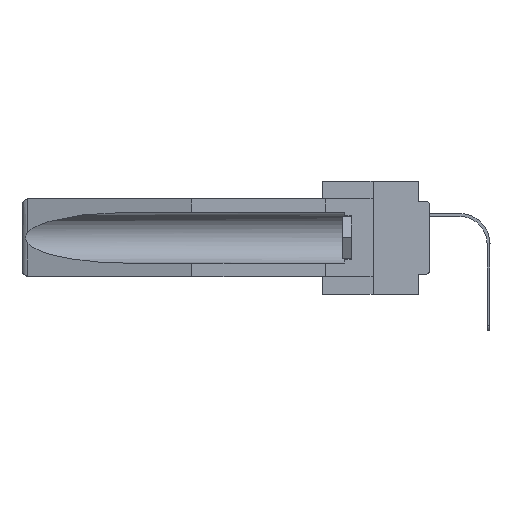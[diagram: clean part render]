
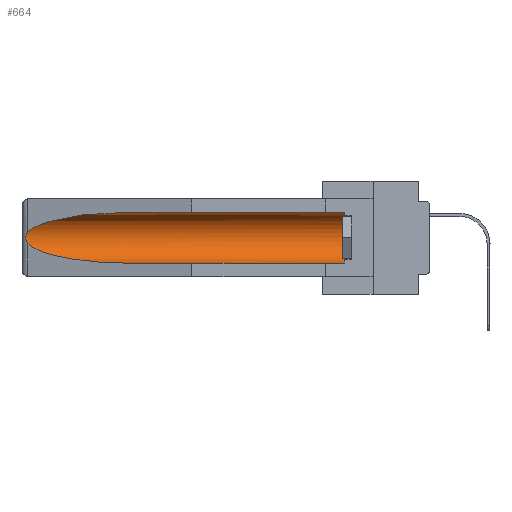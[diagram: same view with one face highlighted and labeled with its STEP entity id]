
A CAD part, left-side view. The second image highlights one B-rep face of the part: STEP entity #664.
In plain terms, the highlighted cylindrical face has radius 2.857 mm (diameter 5.715 mm), a partial arc.
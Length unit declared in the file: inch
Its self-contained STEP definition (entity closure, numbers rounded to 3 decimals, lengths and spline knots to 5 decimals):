
#32 = CARTESIAN_POINT ( 'NONE',  ( 0.155, 1.07973, -0.284 ) ) ;
#664 = ADVANCED_FACE ( 'NONE', ( #27719 ), #1454, .F. ) ;
#842 = CIRCLE ( 'NONE', #33947, 0.1125 ) ;
#1454 = CYLINDRICAL_SURFACE ( 'NONE', #13421, 0.1125 ) ;
#1551 = CARTESIAN_POINT ( 'NONE',  ( 0.26655, 1.53094, -0.18657 ) ) ;
#1882 = CARTESIAN_POINT ( 'NONE',  ( 0.2673, 1.53269, -0.17917 ) ) ;
#3863 = EDGE_CURVE ( 'NONE', #22414, #10565, #8504, .T. ) ;
#3926 = VERTEX_POINT ( 'NONE', #30765 ) ;
#4360 = CARTESIAN_POINT ( 'NONE',  ( 0.21114, 1.30732, -0.059 ) ) ;
#4873 = EDGE_CURVE ( 'NONE', #20516, #3926, #15691, .T. ) ;
#5853 = DIRECTION ( 'NONE',  ( 0., 0., 1. ) ) ;
#6757 = CARTESIAN_POINT ( 'NONE',  ( 0.2675, 1.53308, -0.16763 ) ) ;
#7112 = CARTESIAN_POINT ( 'NONE',  ( 0.155, 1.07973, -0.059 ) ) ;
#7717 = B_SPLINE_CURVE_WITH_KNOTS ( 'NONE', 3,
 ( #20226, #15039, #28470, #30579, #6757, #22804, #1882, #1551, #15196, #12118 ),
 .UNSPECIFIED., .F., .F.,
 ( 4, 2, 2, 2, 4 ),
 ( 0., 0.00029, 0.00058, 0.00087, 0.00117 ),
 .UNSPECIFIED. ) ;
#8137 = CARTESIAN_POINT ( 'NONE',  ( 0.155, 1.07973, -0.059 ) ) ;
#8504 = LINE ( 'NONE', #21622, #13854 ) ;
#8625 = LINE ( 'NONE', #24515, #11952 ) ;
#8847 = ORIENTED_EDGE ( 'NONE', *, *, #4873, .T. ) ;
#9611 = CARTESIAN_POINT ( 'NONE',  ( 0.155, -0.30754, -0.1715 ) ) ;
#10565 = VERTEX_POINT ( 'NONE', #8137 ) ;
#10967 = CARTESIAN_POINT ( 'NONE',  ( 0.155, 0.126, -0.059 ) ) ;
#11381 = DIRECTION ( 'NONE',  ( 0., 1., 0. ) ) ;
#11942 = EDGE_CURVE ( 'NONE', #20156, #20516, #7717, .T. ) ;
#11952 = VECTOR ( 'NONE', #11381, 39.37008 ) ;
#12118 = CARTESIAN_POINT ( 'NONE',  ( 0.26537, 1.52718, -0.19328 ) ) ;
#12153 = EDGE_CURVE ( 'NONE', #31671, #22414, #842, .T. ) ;
#12718 = CARTESIAN_POINT ( 'NONE',  ( 0.26537, 1.52718, -0.14972 ) ) ;
#12835 = CARTESIAN_POINT ( 'NONE',  ( 0.26537, 1.52718, -0.19328 ) ) ;
#13421 = AXIS2_PLACEMENT_3D ( 'NONE', #9611, #22378, #32929 ) ;
#13431 = EDGE_CURVE ( 'NONE', #31671, #3926, #8625, .T. ) ;
#13507 = CARTESIAN_POINT ( 'NONE',  ( 0.25451, 1.48313, -0.24835 ) ) ;
#13854 = VECTOR ( 'NONE', #14033, 39.37008 ) ;
#14033 = DIRECTION ( 'NONE',  ( 0., 1., 0. ) ) ;
#15039 = CARTESIAN_POINT ( 'NONE',  ( 0.26597, 1.52961, -0.15275 ) ) ;
#15196 = CARTESIAN_POINT ( 'NONE',  ( 0.26597, 1.5296, -0.19026 ) ) ;
#15691 =( BOUNDED_CURVE ( )  B_SPLINE_CURVE ( 3, ( #12835, #13507, #29037, #32 ),
 .UNSPECIFIED., .F., .F. ) 
 B_SPLINE_CURVE_WITH_KNOTS ( ( 4, 4 ),
 ( 0.1948, 1.5708 ),
 .UNSPECIFIED. ) 
 CURVE ( )  GEOMETRIC_REPRESENTATION_ITEM ( )  RATIONAL_B_SPLINE_CURVE ( ( 1., 0.848, 0.848, 1. ) ) 
 REPRESENTATION_ITEM ( '' )  );
#16050 = ORIENTED_EDGE ( 'NONE', *, *, #11942, .T. ) ;
#16268 = ORIENTED_EDGE ( 'NONE', *, *, #3863, .T. ) ;
#18728 = ORIENTED_EDGE ( 'NONE', *, *, #13431, .F. ) ;
#19161 = CARTESIAN_POINT ( 'NONE',  ( 0.155, 0.126, -0.1715 ) ) ;
#20156 = VERTEX_POINT ( 'NONE', #12718 ) ;
#20226 = CARTESIAN_POINT ( 'NONE',  ( 0.26537, 1.52718, -0.14972 ) ) ;
#20516 = VERTEX_POINT ( 'NONE', #26438 ) ;
#21377 = CARTESIAN_POINT ( 'NONE',  ( 0.155, 0.126, -0.284 ) ) ;
#21622 = CARTESIAN_POINT ( 'NONE',  ( 0.155, -0.30754, -0.059 ) ) ;
#22254 = DIRECTION ( 'NONE',  ( 0., -1., 0. ) ) ;
#22378 = DIRECTION ( 'NONE',  ( 0., 1., 0. ) ) ;
#22414 = VERTEX_POINT ( 'NONE', #10967 ) ;
#22804 = CARTESIAN_POINT ( 'NONE',  ( 0.2675, 1.53308, -0.17534 ) ) ;
#24515 = CARTESIAN_POINT ( 'NONE',  ( 0.155, -0.30754, -0.284 ) ) ;
#25070 = CARTESIAN_POINT ( 'NONE',  ( 0.25451, 1.48313, -0.09465 ) ) ;
#26046 = ORIENTED_EDGE ( 'NONE', *, *, #29172, .T. ) ;
#26438 = CARTESIAN_POINT ( 'NONE',  ( 0.26537, 1.52718, -0.19328 ) ) ;
#27059 = EDGE_LOOP ( 'NONE', ( #26046, #16050, #8847, #18728, #30888, #16268 ) ) ;
#27719 = FACE_OUTER_BOUND ( 'NONE', #27059, .T. ) ;
#28470 = CARTESIAN_POINT ( 'NONE',  ( 0.26654, 1.53092, -0.15636 ) ) ;
#29037 = CARTESIAN_POINT ( 'NONE',  ( 0.21114, 1.30732, -0.284 ) ) ;
#29172 = EDGE_CURVE ( 'NONE', #10565, #20156, #33337, .T. ) ;
#30579 = CARTESIAN_POINT ( 'NONE',  ( 0.2673, 1.5327, -0.16383 ) ) ;
#30765 = CARTESIAN_POINT ( 'NONE',  ( 0.155, 1.07973, -0.284 ) ) ;
#30888 = ORIENTED_EDGE ( 'NONE', *, *, #12153, .T. ) ;
#31671 = VERTEX_POINT ( 'NONE', #21377 ) ;
#32859 = CARTESIAN_POINT ( 'NONE',  ( 0.26537, 1.52718, -0.14972 ) ) ;
#32929 = DIRECTION ( 'NONE',  ( 0., 0., 1. ) ) ;
#33337 =( BOUNDED_CURVE ( )  B_SPLINE_CURVE ( 3, ( #7112, #4360, #25070, #32859 ),
 .UNSPECIFIED., .F., .F. ) 
 B_SPLINE_CURVE_WITH_KNOTS ( ( 4, 4 ),
 ( 4.71239, 6.08839 ),
 .UNSPECIFIED. ) 
 CURVE ( )  GEOMETRIC_REPRESENTATION_ITEM ( )  RATIONAL_B_SPLINE_CURVE ( ( 1., 0.848, 0.848, 1. ) ) 
 REPRESENTATION_ITEM ( '' )  );
#33947 = AXIS2_PLACEMENT_3D ( 'NONE', #19161, #22254, #5853 ) ;
